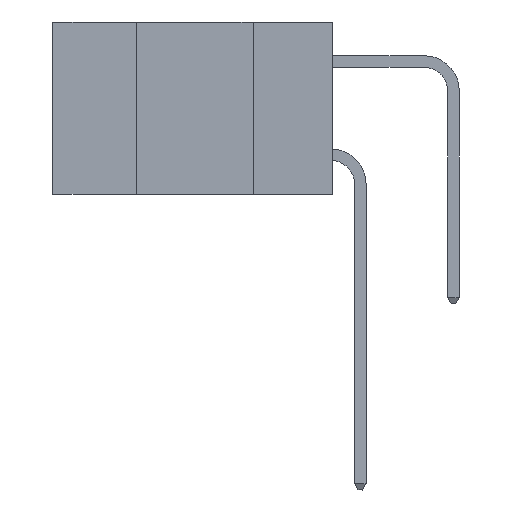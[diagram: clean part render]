
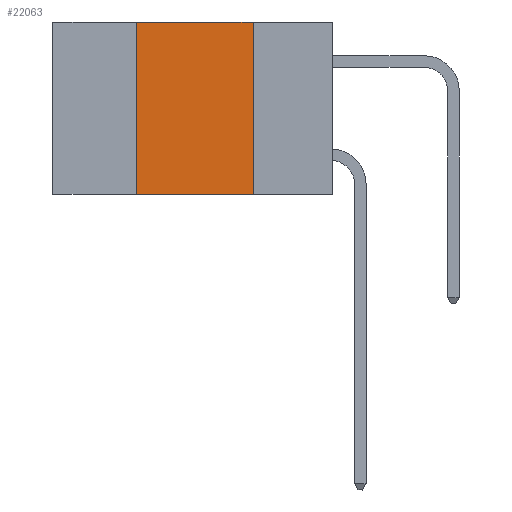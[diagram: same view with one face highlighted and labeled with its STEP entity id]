
A CAD part, left-side view. The second image highlights one B-rep face of the part: STEP entity #22063.
In plain terms, the highlighted planar face has unit normal (-1, 0, 0).
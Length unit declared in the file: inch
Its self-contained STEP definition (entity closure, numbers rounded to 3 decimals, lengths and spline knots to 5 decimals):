
#575 = CARTESIAN_POINT ( 'NONE',  ( 0., 0.42, -0.37 ) ) ;
#1484 = VECTOR ( 'NONE', #17435, 39.37008 ) ;
#1668 = CARTESIAN_POINT ( 'NONE',  ( 0., 0.6, 0. ) ) ;
#2931 = DIRECTION ( 'NONE',  ( 0., -1., 0. ) ) ;
#3054 = CARTESIAN_POINT ( 'NONE',  ( 0., 0.17, 0. ) ) ;
#3168 = LINE ( 'NONE', #23022, #1484 ) ;
#3489 = DIRECTION ( 'NONE',  ( 1., 0., 0. ) ) ;
#4260 = VERTEX_POINT ( 'NONE', #10652 ) ;
#4922 = ORIENTED_EDGE ( 'NONE', *, *, #22875, .F. ) ;
#5009 = EDGE_CURVE ( 'NONE', #22485, #18037, #9706, .T. ) ;
#5035 = AXIS2_PLACEMENT_3D ( 'NONE', #1668, #3489, #5317 ) ;
#5317 = DIRECTION ( 'NONE',  ( 0., 0., -1. ) ) ;
#5998 = CARTESIAN_POINT ( 'NONE',  ( 0., 0.17, 0. ) ) ;
#6016 = FACE_OUTER_BOUND ( 'NONE', #13778, .T. ) ;
#8817 = PLANE ( 'NONE',  #5035 ) ;
#8972 = ORIENTED_EDGE ( 'NONE', *, *, #5009, .F. ) ;
#9634 = VECTOR ( 'NONE', #13748, 39.37008 ) ;
#9706 = LINE ( 'NONE', #5998, #19902 ) ;
#10652 = CARTESIAN_POINT ( 'NONE',  ( 0., 0.42, 0. ) ) ;
#12276 = VERTEX_POINT ( 'NONE', #575 ) ;
#13748 = DIRECTION ( 'NONE',  ( 0., -1., 0. ) ) ;
#13778 = EDGE_LOOP ( 'NONE', ( #8972, #4922, #23395, #21333 ) ) ;
#14093 = EDGE_CURVE ( 'NONE', #12276, #4260, #3168, .T. ) ;
#14134 = EDGE_CURVE ( 'NONE', #12276, #18037, #18135, .T. ) ;
#15816 = CARTESIAN_POINT ( 'NONE',  ( 0., 0.6, -0.37 ) ) ;
#16452 = LINE ( 'NONE', #18930, #20625 ) ;
#17264 = CARTESIAN_POINT ( 'NONE',  ( 0., 0.17, -0.37 ) ) ;
#17435 = DIRECTION ( 'NONE',  ( 0., 0., 1. ) ) ;
#18037 = VERTEX_POINT ( 'NONE', #17264 ) ;
#18135 = LINE ( 'NONE', #15816, #9634 ) ;
#18463 = DIRECTION ( 'NONE',  ( 0., 0., -1. ) ) ;
#18930 = CARTESIAN_POINT ( 'NONE',  ( 0., 0.6, 0. ) ) ;
#19902 = VECTOR ( 'NONE', #18463, 39.37008 ) ;
#20625 = VECTOR ( 'NONE', #2931, 39.37008 ) ;
#21333 = ORIENTED_EDGE ( 'NONE', *, *, #14134, .T. ) ;
#22063 = ADVANCED_FACE ( 'NONE', ( #6016 ), #8817, .F. ) ;
#22485 = VERTEX_POINT ( 'NONE', #3054 ) ;
#22875 = EDGE_CURVE ( 'NONE', #4260, #22485, #16452, .T. ) ;
#23022 = CARTESIAN_POINT ( 'NONE',  ( 0., 0.42, 0. ) ) ;
#23395 = ORIENTED_EDGE ( 'NONE', *, *, #14093, .F. ) ;
